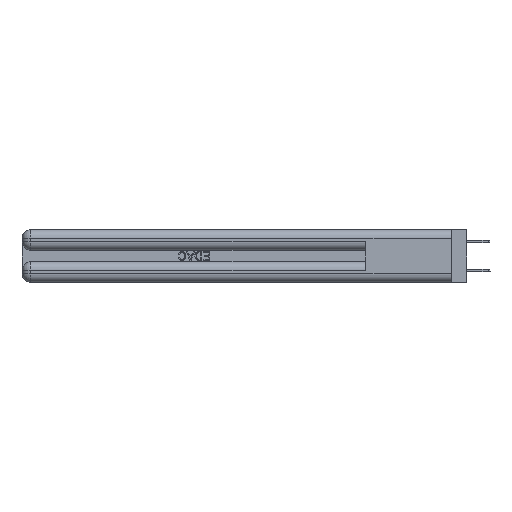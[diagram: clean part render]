
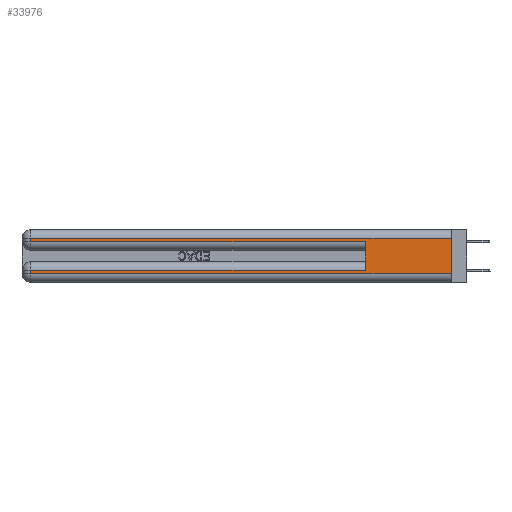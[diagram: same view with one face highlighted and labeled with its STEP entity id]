
A CAD part, left-side view. The second image highlights one B-rep face of the part: STEP entity #33976.
In plain terms, the highlighted planar face has unit normal (-1, 0, 0).
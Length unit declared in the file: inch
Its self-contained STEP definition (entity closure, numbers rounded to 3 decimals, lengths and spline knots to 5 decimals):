
#383 = VECTOR ( 'NONE', #40751, 39.37008 ) ;
#1042 = ORIENTED_EDGE ( 'NONE', *, *, #10448, .T. ) ;
#1096 = VECTOR ( 'NONE', #41618, 39.37008 ) ;
#5271 = VERTEX_POINT ( 'NONE', #25132 ) ;
#5883 = AXIS2_PLACEMENT_3D ( 'NONE', #18243, #31655, #35350 ) ;
#7003 = VECTOR ( 'NONE', #27558, 39.37008 ) ;
#7087 = VERTEX_POINT ( 'NONE', #17474 ) ;
#9945 = VECTOR ( 'NONE', #38247, 39.37008 ) ;
#10101 = VECTOR ( 'NONE', #20250, 39.37008 ) ;
#10448 = EDGE_CURVE ( 'NONE', #23881, #5271, #41186, .T. ) ;
#10663 = LINE ( 'NONE', #33543, #30689 ) ;
#10978 = LINE ( 'NONE', #31732, #383 ) ;
#11059 = EDGE_CURVE ( 'NONE', #23881, #14503, #41145, .T. ) ;
#12410 = ORIENTED_EDGE ( 'NONE', *, *, #30260, .F. ) ;
#12464 = ORIENTED_EDGE ( 'NONE', *, *, #12760, .T. ) ;
#12760 = EDGE_CURVE ( 'NONE', #24851, #16086, #40184, .T. ) ;
#12895 = ORIENTED_EDGE ( 'NONE', *, *, #23768, .T. ) ;
#13307 = VERTEX_POINT ( 'NONE', #22939 ) ;
#13359 = CARTESIAN_POINT ( 'NONE',  ( 0., 0.6, 0.145 ) ) ;
#13363 = VECTOR ( 'NONE', #18854, 39.37008 ) ;
#14503 = VERTEX_POINT ( 'NONE', #19642 ) ;
#14758 = CARTESIAN_POINT ( 'NONE',  ( 0., 0., 0.285 ) ) ;
#16086 = VERTEX_POINT ( 'NONE', #23271 ) ;
#16195 = CARTESIAN_POINT ( 'NONE',  ( 0., 0.6, 0.085 ) ) ;
#17474 = CARTESIAN_POINT ( 'NONE',  ( 0., 2.94, 0.285 ) ) ;
#18243 = CARTESIAN_POINT ( 'NONE',  ( 0., 0., 0.37 ) ) ;
#18854 = DIRECTION ( 'NONE',  ( 0., 1., 0. ) ) ;
#19642 = CARTESIAN_POINT ( 'NONE',  ( 0., 0., 0.06 ) ) ;
#20250 = DIRECTION ( 'NONE',  ( 0., 0., 1. ) ) ;
#20626 = CARTESIAN_POINT ( 'NONE',  ( 0., 0., 0.31 ) ) ;
#21419 = LINE ( 'NONE', #14758, #9945 ) ;
#22939 = CARTESIAN_POINT ( 'NONE',  ( 0., 2.94, 0.06 ) ) ;
#23020 = DIRECTION ( 'NONE',  ( 0., -1., 0. ) ) ;
#23112 = CARTESIAN_POINT ( 'NONE',  ( 0., 2.94, 0.37 ) ) ;
#23271 = CARTESIAN_POINT ( 'NONE',  ( 0., 2.94, 0.085 ) ) ;
#23394 = EDGE_CURVE ( 'NONE', #13307, #14503, #10663, .T. ) ;
#23404 = DIRECTION ( 'NONE',  ( 0., 0., -1. ) ) ;
#23768 = EDGE_CURVE ( 'NONE', #16086, #13307, #24801, .T. ) ;
#23881 = VERTEX_POINT ( 'NONE', #31837 ) ;
#24801 = LINE ( 'NONE', #23112, #37986 ) ;
#24851 = VERTEX_POINT ( 'NONE', #16195 ) ;
#25001 = EDGE_CURVE ( 'NONE', #5271, #7087, #10978, .T. ) ;
#25132 = CARTESIAN_POINT ( 'NONE',  ( 0., 2.94, 0.31 ) ) ;
#25380 = ORIENTED_EDGE ( 'NONE', *, *, #23394, .T. ) ;
#26415 = VERTEX_POINT ( 'NONE', #35297 ) ;
#27389 = LINE ( 'NONE', #13359, #10101 ) ;
#27558 = DIRECTION ( 'NONE',  ( 0., 1., 0. ) ) ;
#27965 = CARTESIAN_POINT ( 'NONE',  ( 0., 0., 0.37 ) ) ;
#28775 = FACE_OUTER_BOUND ( 'NONE', #29464, .T. ) ;
#29464 = EDGE_LOOP ( 'NONE', ( #30589, #1042, #37417, #32935, #12410, #12464, #12895, #25380 ) ) ;
#30260 = EDGE_CURVE ( 'NONE', #24851, #26415, #27389, .T. ) ;
#30589 = ORIENTED_EDGE ( 'NONE', *, *, #11059, .F. ) ;
#30689 = VECTOR ( 'NONE', #23020, 39.37008 ) ;
#31655 = DIRECTION ( 'NONE',  ( 1., 0., 0. ) ) ;
#31732 = CARTESIAN_POINT ( 'NONE',  ( 0., 2.94, 0.37 ) ) ;
#31837 = CARTESIAN_POINT ( 'NONE',  ( 0., 0., 0.31 ) ) ;
#32935 = ORIENTED_EDGE ( 'NONE', *, *, #42682, .T. ) ;
#33543 = CARTESIAN_POINT ( 'NONE',  ( 0., 0., 0.06 ) ) ;
#33976 = ADVANCED_FACE ( 'NONE', ( #28775 ), #42208, .F. ) ;
#35221 = CARTESIAN_POINT ( 'NONE',  ( 0., 0., 0.085 ) ) ;
#35297 = CARTESIAN_POINT ( 'NONE',  ( 0., 0.6, 0.285 ) ) ;
#35350 = DIRECTION ( 'NONE',  ( 0., 0., -1. ) ) ;
#37417 = ORIENTED_EDGE ( 'NONE', *, *, #25001, .T. ) ;
#37986 = VECTOR ( 'NONE', #23404, 39.37008 ) ;
#38247 = DIRECTION ( 'NONE',  ( 0., -1., 0. ) ) ;
#40184 = LINE ( 'NONE', #35221, #13363 ) ;
#40751 = DIRECTION ( 'NONE',  ( 0., 0., -1. ) ) ;
#41145 = LINE ( 'NONE', #27965, #1096 ) ;
#41186 = LINE ( 'NONE', #20626, #7003 ) ;
#41618 = DIRECTION ( 'NONE',  ( 0., 0., -1. ) ) ;
#42208 = PLANE ( 'NONE',  #5883 ) ;
#42682 = EDGE_CURVE ( 'NONE', #7087, #26415, #21419, .T. ) ;
